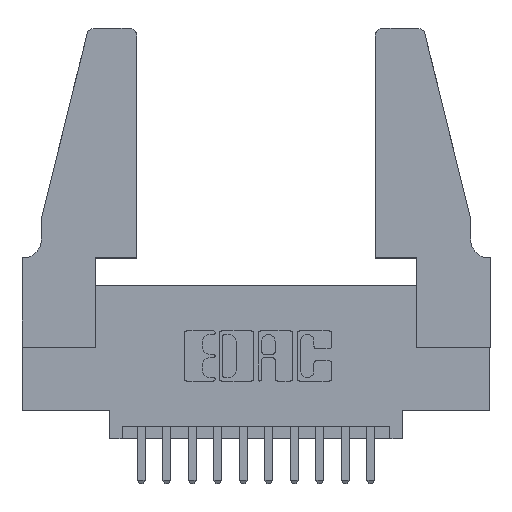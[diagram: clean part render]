
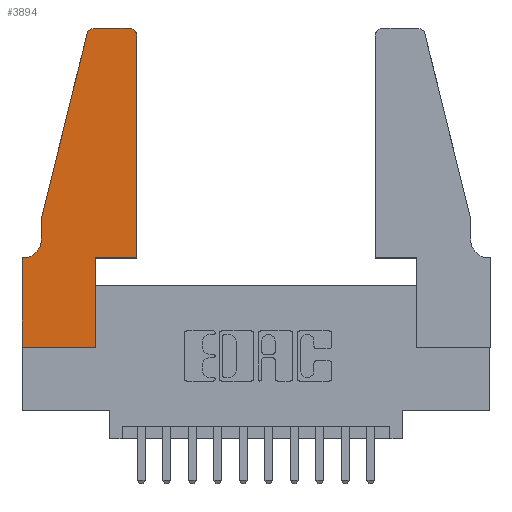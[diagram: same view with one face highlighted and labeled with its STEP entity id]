
A CAD part, top view. The second image highlights one B-rep face of the part: STEP entity #3894.
In plain terms, the highlighted planar face has unit normal (0, 0, 1).
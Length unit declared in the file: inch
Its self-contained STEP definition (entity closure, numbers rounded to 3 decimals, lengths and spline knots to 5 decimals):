
#138 = CARTESIAN_POINT ( 'NONE',  ( 0., 0., 0.37 ) ) ;
#348 = DIRECTION ( 'NONE',  ( 0., -1., 0. ) ) ;
#457 = ORIENTED_EDGE ( 'NONE', *, *, #12898, .T. ) ;
#540 = CARTESIAN_POINT ( 'NONE',  ( 0., 0., 0.37 ) ) ;
#771 = ORIENTED_EDGE ( 'NONE', *, *, #9356, .T. ) ;
#816 = ORIENTED_EDGE ( 'NONE', *, *, #2055, .T. ) ;
#849 = DIRECTION ( 'NONE',  ( 0., 0., 1. ) ) ;
#887 = EDGE_CURVE ( 'NONE', #11603, #9555, #9227, .T. ) ;
#939 = DIRECTION ( 'NONE',  ( 0., 1., 0. ) ) ;
#1124 = VECTOR ( 'NONE', #10669, 39.37008 ) ;
#1126 = CARTESIAN_POINT ( 'NONE',  ( 0.2865, 0.35, 0.37 ) ) ;
#1231 = CARTESIAN_POINT ( 'NONE',  ( 0., 0., 0.37 ) ) ;
#1243 = EDGE_CURVE ( 'NONE', #4578, #4039, #13445, .T. ) ;
#1244 = VECTOR ( 'NONE', #939, 39.37008 ) ;
#1494 = DIRECTION ( 'NONE',  ( -1., 0., 0. ) ) ;
#1539 = EDGE_LOOP ( 'NONE', ( #8128, #11326, #2266, #14242, #771, #5583, #11036, #11381, #4239, #457, #10246, #816 ) ) ;
#1796 = EDGE_CURVE ( 'NONE', #12721, #8892, #4644, .T. ) ;
#2017 = DIRECTION ( 'NONE',  ( 0., 0., -1. ) ) ;
#2055 = EDGE_CURVE ( 'NONE', #8892, #4578, #8505, .T. ) ;
#2140 = EDGE_CURVE ( 'NONE', #12103, #6303, #3747, .T. ) ;
#2266 = ORIENTED_EDGE ( 'NONE', *, *, #887, .T. ) ;
#2369 = CARTESIAN_POINT ( 'NONE',  ( 0.4205, 1.25, 0.37 ) ) ;
#2901 = LINE ( 'NONE', #3600, #5702 ) ;
#3229 = CARTESIAN_POINT ( 'NONE',  ( 0.0755, 0.5, 0.37 ) ) ;
#3311 = CARTESIAN_POINT ( 'NONE',  ( 0.4205, 1.22, 0.37 ) ) ;
#3565 = CARTESIAN_POINT ( 'NONE',  ( 0.4505, 0.35, 0.37 ) ) ;
#3577 = DIRECTION ( 'NONE',  ( 1., 0., 0. ) ) ;
#3600 = CARTESIAN_POINT ( 'NONE',  ( 0.0755, 0.5, 0.37 ) ) ;
#3747 = LINE ( 'NONE', #1231, #9371 ) ;
#3778 = CARTESIAN_POINT ( 'NONE',  ( 0.2865, 0., 0.37 ) ) ;
#3840 = LINE ( 'NONE', #138, #12975 ) ;
#3894 = ADVANCED_FACE ( 'NONE', ( #5730 ), #12510, .T. ) ;
#4039 = VERTEX_POINT ( 'NONE', #13180 ) ;
#4239 = ORIENTED_EDGE ( 'NONE', *, *, #12994, .T. ) ;
#4407 = VERTEX_POINT ( 'NONE', #7928 ) ;
#4578 = VERTEX_POINT ( 'NONE', #2369 ) ;
#4644 = LINE ( 'NONE', #11803, #1124 ) ;
#5022 = AXIS2_PLACEMENT_3D ( 'NONE', #13699, #10311, #13751 ) ;
#5313 = CARTESIAN_POINT ( 'NONE',  ( 0.0055, 0.42, 0.37 ) ) ;
#5583 = ORIENTED_EDGE ( 'NONE', *, *, #11418, .T. ) ;
#5702 = VECTOR ( 'NONE', #348, 39.37008 ) ;
#5730 = FACE_OUTER_BOUND ( 'NONE', #1539, .T. ) ;
#5785 = CARTESIAN_POINT ( 'NONE',  ( 0., 0.35, 0.37 ) ) ;
#5869 = CARTESIAN_POINT ( 'NONE',  ( 0.4505, 0.35, 0.37 ) ) ;
#5916 = DIRECTION ( 'NONE',  ( 1., 0., 0. ) ) ;
#5996 = LINE ( 'NONE', #5869, #12486 ) ;
#6119 = CARTESIAN_POINT ( 'NONE',  ( 0., 0.35, 0.37 ) ) ;
#6246 = VECTOR ( 'NONE', #14429, 39.37008 ) ;
#6303 = VERTEX_POINT ( 'NONE', #3778 ) ;
#6599 = AXIS2_PLACEMENT_3D ( 'NONE', #5313, #2017, #7488 ) ;
#7488 = DIRECTION ( 'NONE',  ( -1., 0., 0. ) ) ;
#7715 = DIRECTION ( 'NONE',  ( 1., 0., 0. ) ) ;
#7865 = DIRECTION ( 'NONE',  ( 1., 0., 0. ) ) ;
#7928 = CARTESIAN_POINT ( 'NONE',  ( 0.0055, 0.35, 0.37 ) ) ;
#8086 = DIRECTION ( 'NONE',  ( 0., 0., 1. ) ) ;
#8128 = ORIENTED_EDGE ( 'NONE', *, *, #1243, .T. ) ;
#8256 = CARTESIAN_POINT ( 'NONE',  ( 0.4505, 1.22, 0.37 ) ) ;
#8287 = VERTEX_POINT ( 'NONE', #9048 ) ;
#8406 = CIRCLE ( 'NONE', #6599, 0.07 ) ;
#8505 = CIRCLE ( 'NONE', #10150, 0.03 ) ;
#8517 = CARTESIAN_POINT ( 'NONE',  ( 0.0755, 0.5, 0.37 ) ) ;
#8892 = VERTEX_POINT ( 'NONE', #8256 ) ;
#9048 = CARTESIAN_POINT ( 'NONE',  ( 0.0755, 0.42, 0.37 ) ) ;
#9227 = LINE ( 'NONE', #3229, #13103 ) ;
#9356 = EDGE_CURVE ( 'NONE', #8287, #4407, #8406, .T. ) ;
#9371 = VECTOR ( 'NONE', #7865, 39.37008 ) ;
#9555 = VERTEX_POINT ( 'NONE', #8517 ) ;
#10150 = AXIS2_PLACEMENT_3D ( 'NONE', #3311, #849, #7715 ) ;
#10246 = ORIENTED_EDGE ( 'NONE', *, *, #1796, .T. ) ;
#10311 = DIRECTION ( 'NONE',  ( 0., 0., 1. ) ) ;
#10451 = VECTOR ( 'NONE', #1494, 39.37008 ) ;
#10627 = CIRCLE ( 'NONE', #5022, 0.03 ) ;
#10669 = DIRECTION ( 'NONE',  ( 0., 1., 0. ) ) ;
#10684 = CARTESIAN_POINT ( 'NONE',  ( 0.2605, 1.25, 0.37 ) ) ;
#11036 = ORIENTED_EDGE ( 'NONE', *, *, #14414, .T. ) ;
#11101 = EDGE_CURVE ( 'NONE', #4039, #11603, #10627, .T. ) ;
#11250 = EDGE_CURVE ( 'NONE', #9555, #8287, #2901, .T. ) ;
#11326 = ORIENTED_EDGE ( 'NONE', *, *, #11101, .T. ) ;
#11381 = ORIENTED_EDGE ( 'NONE', *, *, #2140, .T. ) ;
#11418 = EDGE_CURVE ( 'NONE', #4407, #12067, #12731, .T. ) ;
#11603 = VERTEX_POINT ( 'NONE', #13663 ) ;
#11803 = CARTESIAN_POINT ( 'NONE',  ( 0.4505, 0.35, 0.37 ) ) ;
#12067 = VERTEX_POINT ( 'NONE', #6119 ) ;
#12103 = VERTEX_POINT ( 'NONE', #540 ) ;
#12129 = CARTESIAN_POINT ( 'NONE',  ( 0.2865, 0.35, 0.37 ) ) ;
#12486 = VECTOR ( 'NONE', #5916, 39.37008 ) ;
#12510 = PLANE ( 'NONE',  #14051 ) ;
#12627 = VERTEX_POINT ( 'NONE', #12129 ) ;
#12721 = VERTEX_POINT ( 'NONE', #3565 ) ;
#12731 = LINE ( 'NONE', #13173, #6246 ) ;
#12898 = EDGE_CURVE ( 'NONE', #12627, #12721, #5996, .T. ) ;
#12975 = VECTOR ( 'NONE', #13459, 39.37008 ) ;
#12994 = EDGE_CURVE ( 'NONE', #6303, #12627, #13366, .T. ) ;
#13103 = VECTOR ( 'NONE', #13440, 39.37008 ) ;
#13173 = CARTESIAN_POINT ( 'NONE',  ( 0.0755, 0.35, 0.37 ) ) ;
#13180 = CARTESIAN_POINT ( 'NONE',  ( 0.284, 1.25, 0.37 ) ) ;
#13366 = LINE ( 'NONE', #1126, #1244 ) ;
#13440 = DIRECTION ( 'NONE',  ( -0.239, -0.971, 0. ) ) ;
#13445 = LINE ( 'NONE', #10684, #10451 ) ;
#13459 = DIRECTION ( 'NONE',  ( 0., -1., 0. ) ) ;
#13663 = CARTESIAN_POINT ( 'NONE',  ( 0.25487, 1.22718, 0.37 ) ) ;
#13699 = CARTESIAN_POINT ( 'NONE',  ( 0.284, 1.22, 0.37 ) ) ;
#13751 = DIRECTION ( 'NONE',  ( 1., 0., 0. ) ) ;
#14051 = AXIS2_PLACEMENT_3D ( 'NONE', #5785, #8086, #3577 ) ;
#14242 = ORIENTED_EDGE ( 'NONE', *, *, #11250, .T. ) ;
#14414 = EDGE_CURVE ( 'NONE', #12067, #12103, #3840, .T. ) ;
#14429 = DIRECTION ( 'NONE',  ( -1., 0., 0. ) ) ;
